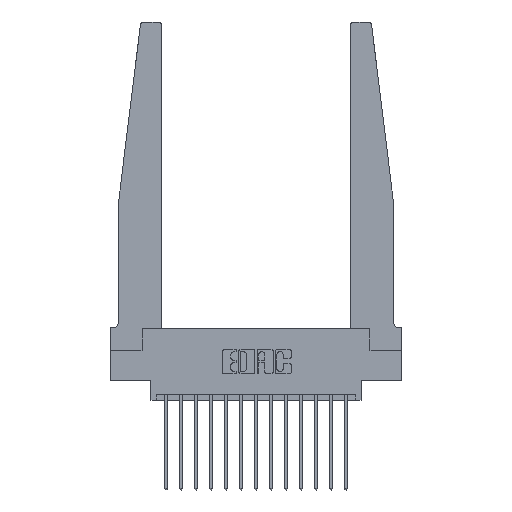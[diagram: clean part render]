
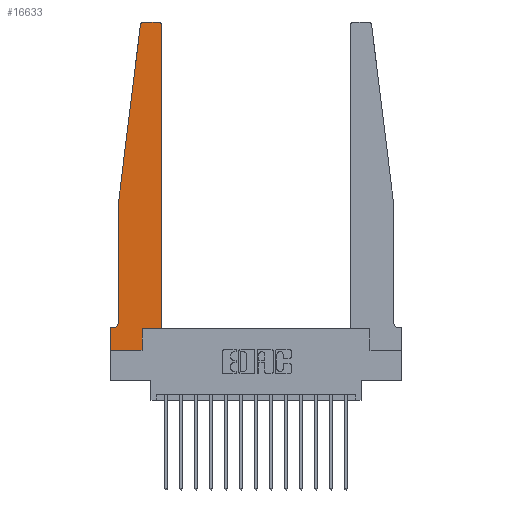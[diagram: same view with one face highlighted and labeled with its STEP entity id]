
A CAD part, top view. The second image highlights one B-rep face of the part: STEP entity #16633.
In plain terms, the highlighted planar face has unit normal (0, 0, 1).
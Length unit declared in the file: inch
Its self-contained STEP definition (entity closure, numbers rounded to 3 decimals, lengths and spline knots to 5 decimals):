
#4 = VECTOR ( 'NONE', #2464, 39.37008 ) ;
#55 = VERTEX_POINT ( 'NONE', #6930 ) ;
#254 = CARTESIAN_POINT ( 'NONE',  ( 0.27653, 2.72, 0.37 ) ) ;
#309 = CARTESIAN_POINT ( 'NONE',  ( 0.425, 0.18, 0.37 ) ) ;
#511 = CARTESIAN_POINT ( 'NONE',  ( 0.065, 0.1875, 0.37 ) ) ;
#583 = DIRECTION ( 'NONE',  ( -1., 0., 0. ) ) ;
#840 = ORIENTED_EDGE ( 'NONE', *, *, #6984, .T. ) ;
#1046 = EDGE_CURVE ( 'NONE', #14240, #9045, #3136, .T. ) ;
#1052 = DIRECTION ( 'NONE',  ( 1., 0., 0. ) ) ;
#1662 = VECTOR ( 'NONE', #3707, 39.37008 ) ;
#1933 = ORIENTED_EDGE ( 'NONE', *, *, #16836, .T. ) ;
#2449 = VERTEX_POINT ( 'NONE', #11614 ) ;
#2459 = EDGE_CURVE ( 'NONE', #55, #5507, #8718, .T. ) ;
#2464 = DIRECTION ( 'NONE',  ( 1., 0., 0. ) ) ;
#2468 = CARTESIAN_POINT ( 'NONE',  ( 0.27653, 2.75, 0.37 ) ) ;
#2493 = DIRECTION ( 'NONE',  ( 0., 0., 1. ) ) ;
#2536 = CARTESIAN_POINT ( 'NONE',  ( 0.2605, 0., 0.37 ) ) ;
#2629 = ORIENTED_EDGE ( 'NONE', *, *, #8011, .T. ) ;
#2932 = AXIS2_PLACEMENT_3D ( 'NONE', #7758, #4730, #11647 ) ;
#3136 = LINE ( 'NONE', #12745, #17362 ) ;
#3226 = VERTEX_POINT ( 'NONE', #5593 ) ;
#3290 = DIRECTION ( 'NONE',  ( -1., 0., 0. ) ) ;
#3463 = VERTEX_POINT ( 'NONE', #9817 ) ;
#3491 = VERTEX_POINT ( 'NONE', #11136 ) ;
#3563 = PLANE ( 'NONE',  #2932 ) ;
#3707 = DIRECTION ( 'NONE',  ( -0.122, -0.992, 0. ) ) ;
#3713 = DIRECTION ( 'NONE',  ( 0., 1., 0. ) ) ;
#3810 = CIRCLE ( 'NONE', #11846, 0.05 ) ;
#3821 = CARTESIAN_POINT ( 'NONE',  ( 0.395, 2.72, 0.37 ) ) ;
#4012 = VECTOR ( 'NONE', #583, 39.37008 ) ;
#4080 = DIRECTION ( 'NONE',  ( -1., 0., 0. ) ) ;
#4730 = DIRECTION ( 'NONE',  ( 0., 0., 1. ) ) ;
#5116 = CARTESIAN_POINT ( 'NONE',  ( 0.065, 1.25, 0.37 ) ) ;
#5454 = CARTESIAN_POINT ( 'NONE',  ( 0., 0., 0.37 ) ) ;
#5507 = VERTEX_POINT ( 'NONE', #2468 ) ;
#5516 = LINE ( 'NONE', #5116, #1662 ) ;
#5593 = CARTESIAN_POINT ( 'NONE',  ( 0.425, 2.72, 0.37 ) ) ;
#6095 = DIRECTION ( 'NONE',  ( 1., 0., 0. ) ) ;
#6502 = ORIENTED_EDGE ( 'NONE', *, *, #14277, .T. ) ;
#6795 = CARTESIAN_POINT ( 'NONE',  ( 0.2605, 0.18, 0.37 ) ) ;
#6799 = EDGE_CURVE ( 'NONE', #3463, #3226, #14373, .T. ) ;
#6835 = VECTOR ( 'NONE', #3290, 39.37008 ) ;
#6860 = VERTEX_POINT ( 'NONE', #17623 ) ;
#6930 = CARTESIAN_POINT ( 'NONE',  ( 0.395, 2.75, 0.37 ) ) ;
#6984 = EDGE_CURVE ( 'NONE', #14099, #3463, #15723, .T. ) ;
#7075 = AXIS2_PLACEMENT_3D ( 'NONE', #254, #15261, #16419 ) ;
#7484 = VECTOR ( 'NONE', #7831, 39.37008 ) ;
#7698 = CARTESIAN_POINT ( 'NONE',  ( 0.2605, 0.18, 0.37 ) ) ;
#7758 = CARTESIAN_POINT ( 'NONE',  ( 0., 0.1875, 0.37 ) ) ;
#7794 = CARTESIAN_POINT ( 'NONE',  ( 0.425, 0.18, 0.37 ) ) ;
#7831 = DIRECTION ( 'NONE',  ( 0., -1., 0. ) ) ;
#7885 = VECTOR ( 'NONE', #8126, 39.37008 ) ;
#8011 = EDGE_CURVE ( 'NONE', #9045, #14099, #10771, .T. ) ;
#8126 = DIRECTION ( 'NONE',  ( 0., 1., 0. ) ) ;
#8282 = CARTESIAN_POINT ( 'NONE',  ( 0.065, 1.25, 0.37 ) ) ;
#8296 = ORIENTED_EDGE ( 'NONE', *, *, #6799, .T. ) ;
#8718 = LINE ( 'NONE', #14183, #4012 ) ;
#8948 = EDGE_CURVE ( 'NONE', #3491, #12956, #5516, .T. ) ;
#9045 = VERTEX_POINT ( 'NONE', #2536 ) ;
#9291 = EDGE_CURVE ( 'NONE', #14453, #2449, #17013, .T. ) ;
#9311 = CARTESIAN_POINT ( 'NONE',  ( 0.015, 0.1875, 0.37 ) ) ;
#9555 = CARTESIAN_POINT ( 'NONE',  ( 0.015, 0.2375, 0.37 ) ) ;
#9817 = CARTESIAN_POINT ( 'NONE',  ( 0.425, 0.18, 0.37 ) ) ;
#10546 = EDGE_LOOP ( 'NONE', ( #13013, #6502, #11598, #1933, #15706, #17707, #11359, #14813, #2629, #840, #8296, #10818 ) ) ;
#10567 = LINE ( 'NONE', #16029, #7484 ) ;
#10771 = LINE ( 'NONE', #6795, #7885 ) ;
#10818 = ORIENTED_EDGE ( 'NONE', *, *, #16097, .T. ) ;
#11136 = CARTESIAN_POINT ( 'NONE',  ( 0.24675, 2.72367, 0.37 ) ) ;
#11359 = ORIENTED_EDGE ( 'NONE', *, *, #12652, .T. ) ;
#11598 = ORIENTED_EDGE ( 'NONE', *, *, #8948, .T. ) ;
#11614 = CARTESIAN_POINT ( 'NONE',  ( 0., 0.1875, 0.37 ) ) ;
#11647 = DIRECTION ( 'NONE',  ( 1., 0., 0. ) ) ;
#11846 = AXIS2_PLACEMENT_3D ( 'NONE', #9555, #16542, #4080 ) ;
#12133 = VECTOR ( 'NONE', #3713, 39.37008 ) ;
#12652 = EDGE_CURVE ( 'NONE', #2449, #14240, #10567, .T. ) ;
#12745 = CARTESIAN_POINT ( 'NONE',  ( 0., 0., 0.37 ) ) ;
#12956 = VERTEX_POINT ( 'NONE', #8282 ) ;
#13013 = ORIENTED_EDGE ( 'NONE', *, *, #2459, .T. ) ;
#13247 = VECTOR ( 'NONE', #17467, 39.37008 ) ;
#13606 = CARTESIAN_POINT ( 'NONE',  ( 0.065, 1.25, 0.37 ) ) ;
#14099 = VERTEX_POINT ( 'NONE', #7698 ) ;
#14183 = CARTESIAN_POINT ( 'NONE',  ( 0.25, 2.75, 0.37 ) ) ;
#14240 = VERTEX_POINT ( 'NONE', #5454 ) ;
#14277 = EDGE_CURVE ( 'NONE', #5507, #3491, #14832, .T. ) ;
#14373 = LINE ( 'NONE', #309, #12133 ) ;
#14453 = VERTEX_POINT ( 'NONE', #9311 ) ;
#14775 = LINE ( 'NONE', #13606, #13247 ) ;
#14813 = ORIENTED_EDGE ( 'NONE', *, *, #1046, .T. ) ;
#14832 = CIRCLE ( 'NONE', #7075, 0.03 ) ;
#15261 = DIRECTION ( 'NONE',  ( 0., 0., 1. ) ) ;
#15706 = ORIENTED_EDGE ( 'NONE', *, *, #17248, .T. ) ;
#15723 = LINE ( 'NONE', #7794, #4 ) ;
#16029 = CARTESIAN_POINT ( 'NONE',  ( 0., 0., 0.37 ) ) ;
#16097 = EDGE_CURVE ( 'NONE', #3226, #55, #16703, .T. ) ;
#16147 = AXIS2_PLACEMENT_3D ( 'NONE', #3821, #2493, #1052 ) ;
#16419 = DIRECTION ( 'NONE',  ( 1., 0., 0. ) ) ;
#16542 = DIRECTION ( 'NONE',  ( 0., 0., -1. ) ) ;
#16633 = ADVANCED_FACE ( 'NONE', ( #17203 ), #3563, .T. ) ;
#16703 = CIRCLE ( 'NONE', #16147, 0.03 ) ;
#16836 = EDGE_CURVE ( 'NONE', #12956, #6860, #14775, .T. ) ;
#17013 = LINE ( 'NONE', #511, #6835 ) ;
#17203 = FACE_OUTER_BOUND ( 'NONE', #10546, .T. ) ;
#17248 = EDGE_CURVE ( 'NONE', #6860, #14453, #3810, .T. ) ;
#17362 = VECTOR ( 'NONE', #6095, 39.37008 ) ;
#17467 = DIRECTION ( 'NONE',  ( 0., -1., 0. ) ) ;
#17623 = CARTESIAN_POINT ( 'NONE',  ( 0.065, 0.2375, 0.37 ) ) ;
#17707 = ORIENTED_EDGE ( 'NONE', *, *, #9291, .T. ) ;
